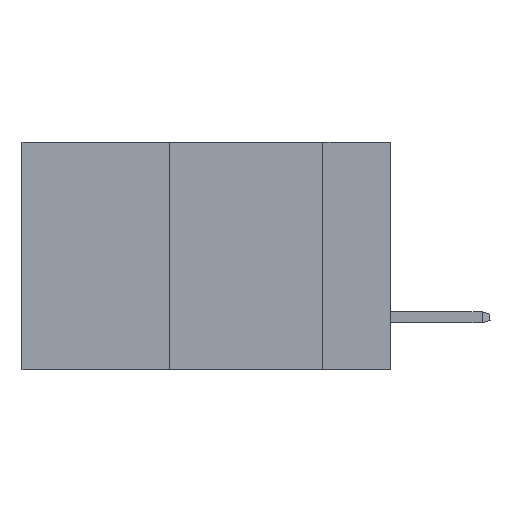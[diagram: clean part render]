
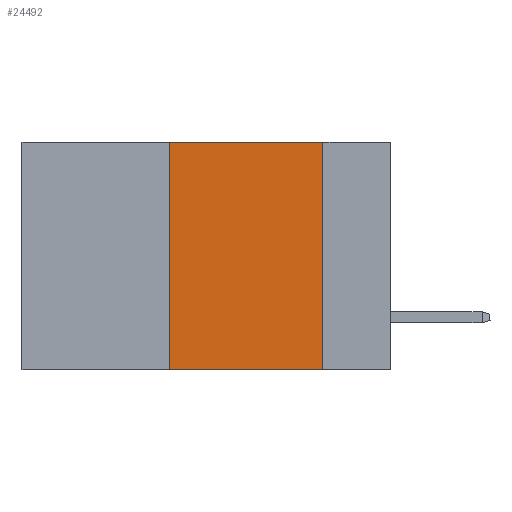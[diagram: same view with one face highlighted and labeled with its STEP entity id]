
A CAD part, left-side view. The second image highlights one B-rep face of the part: STEP entity #24492.
In plain terms, the highlighted planar face has unit normal (-1, 0, 0).
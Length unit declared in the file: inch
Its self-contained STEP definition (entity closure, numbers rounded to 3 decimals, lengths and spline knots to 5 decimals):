
#898 = DIRECTION ( 'NONE',  ( 0., -1., 0. ) ) ;
#1243 = VERTEX_POINT ( 'NONE', #1836 ) ;
#1836 = CARTESIAN_POINT ( 'NONE',  ( 0., 0.11, 0. ) ) ;
#2002 = LINE ( 'NONE', #34480, #22859 ) ;
#2484 = EDGE_CURVE ( 'NONE', #4331, #1243, #5431, .T. ) ;
#3305 = DIRECTION ( 'NONE',  ( 0., -1., 0. ) ) ;
#3639 = EDGE_CURVE ( 'NONE', #48588, #4331, #8340, .T. ) ;
#4331 = VERTEX_POINT ( 'NONE', #7084 ) ;
#5122 = CARTESIAN_POINT ( 'NONE',  ( 0., 0.6, 0. ) ) ;
#5431 = LINE ( 'NONE', #5122, #32872 ) ;
#5927 = CARTESIAN_POINT ( 'NONE',  ( 0., 0.11, -0.37 ) ) ;
#5937 = EDGE_CURVE ( 'NONE', #1243, #46076, #2002, .T. ) ;
#6512 = VECTOR ( 'NONE', #898, 39.37008 ) ;
#7084 = CARTESIAN_POINT ( 'NONE',  ( 0., 0.36, 0. ) ) ;
#7148 = VECTOR ( 'NONE', #21938, 39.37008 ) ;
#8340 = LINE ( 'NONE', #18592, #7148 ) ;
#8865 = CARTESIAN_POINT ( 'NONE',  ( 0., 0.6, -0.37 ) ) ;
#11382 = EDGE_LOOP ( 'NONE', ( #46711, #28074, #11472, #12205 ) ) ;
#11472 = ORIENTED_EDGE ( 'NONE', *, *, #3639, .F. ) ;
#12205 = ORIENTED_EDGE ( 'NONE', *, *, #37657, .T. ) ;
#12297 = DIRECTION ( 'NONE',  ( 1., 0., 0. ) ) ;
#15133 = AXIS2_PLACEMENT_3D ( 'NONE', #24323, #12297, #28109 ) ;
#18592 = CARTESIAN_POINT ( 'NONE',  ( 0., 0.36, 0. ) ) ;
#20501 = PLANE ( 'NONE',  #15133 ) ;
#21938 = DIRECTION ( 'NONE',  ( 0., 0., 1. ) ) ;
#22859 = VECTOR ( 'NONE', #34322, 39.37008 ) ;
#24323 = CARTESIAN_POINT ( 'NONE',  ( 0., 0.6, 0. ) ) ;
#24492 = ADVANCED_FACE ( 'NONE', ( #25778 ), #20501, .F. ) ;
#25778 = FACE_OUTER_BOUND ( 'NONE', #11382, .T. ) ;
#28074 = ORIENTED_EDGE ( 'NONE', *, *, #2484, .F. ) ;
#28109 = DIRECTION ( 'NONE',  ( 0., 0., -1. ) ) ;
#32140 = LINE ( 'NONE', #8865, #6512 ) ;
#32872 = VECTOR ( 'NONE', #3305, 39.37008 ) ;
#34322 = DIRECTION ( 'NONE',  ( 0., 0., -1. ) ) ;
#34480 = CARTESIAN_POINT ( 'NONE',  ( 0., 0.11, 0. ) ) ;
#37657 = EDGE_CURVE ( 'NONE', #48588, #46076, #32140, .T. ) ;
#39735 = CARTESIAN_POINT ( 'NONE',  ( 0., 0.36, -0.37 ) ) ;
#46076 = VERTEX_POINT ( 'NONE', #5927 ) ;
#46711 = ORIENTED_EDGE ( 'NONE', *, *, #5937, .F. ) ;
#48588 = VERTEX_POINT ( 'NONE', #39735 ) ;
